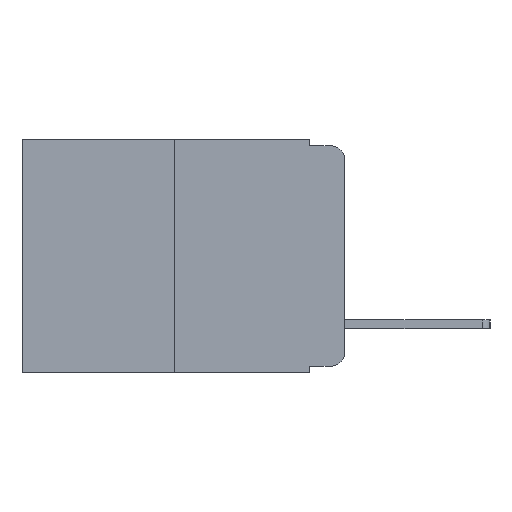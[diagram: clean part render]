
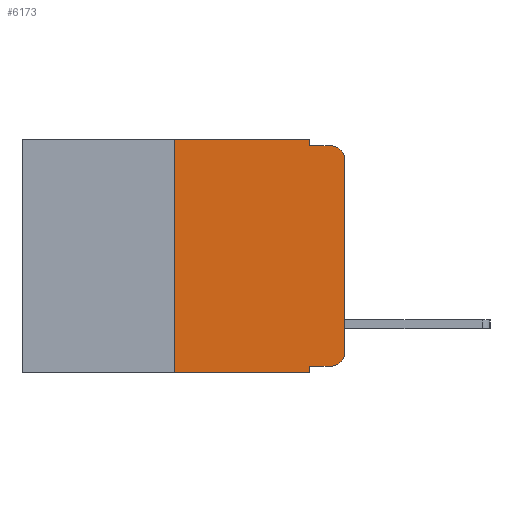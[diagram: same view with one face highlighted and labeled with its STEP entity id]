
A CAD part, left-side view. The second image highlights one B-rep face of the part: STEP entity #6173.
In plain terms, the highlighted planar face has unit normal (-1, 0, 0).
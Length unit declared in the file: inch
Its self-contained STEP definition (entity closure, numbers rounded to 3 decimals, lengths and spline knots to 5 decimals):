
#895 = LINE ( 'NONE', #17830, #14827 ) ;
#1033 = ORIENTED_EDGE ( 'NONE', *, *, #17482, .F. ) ;
#1414 = VERTEX_POINT ( 'NONE', #18648 ) ;
#1776 = EDGE_LOOP ( 'NONE', ( #20185, #4307, #9606, #12827, #3194, #1033, #14149, #10768, #17269, #14955 ) ) ;
#3194 = ORIENTED_EDGE ( 'NONE', *, *, #20132, .F. ) ;
#3628 = DIRECTION ( 'NONE',  ( -1., 0., 0. ) ) ;
#3835 = DIRECTION ( 'NONE',  ( 0., -1., 0. ) ) ;
#4049 = CARTESIAN_POINT ( 'NONE',  ( 0., 0.051, 0. ) ) ;
#4067 = VERTEX_POINT ( 'NONE', #14452 ) ;
#4307 = ORIENTED_EDGE ( 'NONE', *, *, #20642, .T. ) ;
#4696 = VERTEX_POINT ( 'NONE', #22398 ) ;
#4763 = CARTESIAN_POINT ( 'NONE',  ( 0., 0.473, 0. ) ) ;
#5583 = DIRECTION ( 'NONE',  ( 0., 0., 1. ) ) ;
#5677 = VECTOR ( 'NONE', #7814, 39.37008 ) ;
#5726 = CARTESIAN_POINT ( 'NONE',  ( 0., 0.02, -0.03 ) ) ;
#5925 = CARTESIAN_POINT ( 'NONE',  ( 0., 0.051, -0.01 ) ) ;
#6173 = ADVANCED_FACE ( 'NONE', ( #21610 ), #21680, .F. ) ;
#6362 = CARTESIAN_POINT ( 'NONE',  ( 0., 0.051, 0. ) ) ;
#6380 = AXIS2_PLACEMENT_3D ( 'NONE', #14364, #3628, #16050 ) ;
#6572 = VECTOR ( 'NONE', #11750, 39.37008 ) ;
#7038 = VECTOR ( 'NONE', #21076, 39.37008 ) ;
#7577 = DIRECTION ( 'NONE',  ( 0., 0., -1. ) ) ;
#7814 = DIRECTION ( 'NONE',  ( 0., 0., -1. ) ) ;
#8091 = CARTESIAN_POINT ( 'NONE',  ( 0., 0.25, 0. ) ) ;
#8227 = VERTEX_POINT ( 'NONE', #16112 ) ;
#8401 = CIRCLE ( 'NONE', #6380, 0.02 ) ;
#9240 = DIRECTION ( 'NONE',  ( 0., -1., 0. ) ) ;
#9606 = ORIENTED_EDGE ( 'NONE', *, *, #19578, .F. ) ;
#9903 = VECTOR ( 'NONE', #3835, 39.37008 ) ;
#10152 = CARTESIAN_POINT ( 'NONE',  ( 0., 0.051, 0. ) ) ;
#10335 = LINE ( 'NONE', #11025, #13747 ) ;
#10343 = CARTESIAN_POINT ( 'NONE',  ( 0., 0.473, 0. ) ) ;
#10585 = LINE ( 'NONE', #4049, #5677 ) ;
#10768 = ORIENTED_EDGE ( 'NONE', *, *, #16415, .F. ) ;
#11025 = CARTESIAN_POINT ( 'NONE',  ( 0., 0.25, 0. ) ) ;
#11102 = EDGE_CURVE ( 'NONE', #8227, #12383, #14393, .T. ) ;
#11103 = CARTESIAN_POINT ( 'NONE',  ( 0., 0.051, -0.01 ) ) ;
#11256 = DIRECTION ( 'NONE',  ( 0., -1., 0. ) ) ;
#11750 = DIRECTION ( 'NONE',  ( 0., 0., -1. ) ) ;
#12000 = DIRECTION ( 'NONE',  ( 1., 0., 0. ) ) ;
#12383 = VERTEX_POINT ( 'NONE', #18413 ) ;
#12389 = LINE ( 'NONE', #11103, #16309 ) ;
#12827 = ORIENTED_EDGE ( 'NONE', *, *, #18543, .F. ) ;
#13037 = EDGE_CURVE ( 'NONE', #4696, #4067, #8401, .T. ) ;
#13095 = AXIS2_PLACEMENT_3D ( 'NONE', #5726, #17793, #7577 ) ;
#13642 = DIRECTION ( 'NONE',  ( 0., -1., 0. ) ) ;
#13747 = VECTOR ( 'NONE', #5583, 39.37008 ) ;
#13942 = LINE ( 'NONE', #10343, #19256 ) ;
#14149 = ORIENTED_EDGE ( 'NONE', *, *, #11102, .T. ) ;
#14364 = CARTESIAN_POINT ( 'NONE',  ( 0., 0.02, -0.313 ) ) ;
#14393 = LINE ( 'NONE', #22484, #9903 ) ;
#14452 = CARTESIAN_POINT ( 'NONE',  ( 0., 0., -0.313 ) ) ;
#14751 = VERTEX_POINT ( 'NONE', #10152 ) ;
#14827 = VECTOR ( 'NONE', #11256, 39.37008 ) ;
#14843 = AXIS2_PLACEMENT_3D ( 'NONE', #4763, #12000, #18508 ) ;
#14955 = ORIENTED_EDGE ( 'NONE', *, *, #13037, .T. ) ;
#15212 = VERTEX_POINT ( 'NONE', #20862 ) ;
#15319 = EDGE_CURVE ( 'NONE', #22391, #4696, #895, .T. ) ;
#15381 = VERTEX_POINT ( 'NONE', #5925 ) ;
#15568 = VERTEX_POINT ( 'NONE', #8091 ) ;
#15735 = LINE ( 'NONE', #19416, #7038 ) ;
#16012 = CIRCLE ( 'NONE', #13095, 0.02 ) ;
#16050 = DIRECTION ( 'NONE',  ( 0., 0., -1. ) ) ;
#16112 = CARTESIAN_POINT ( 'NONE',  ( 0., 0.25, -0.343 ) ) ;
#16309 = VECTOR ( 'NONE', #9240, 39.37008 ) ;
#16415 = EDGE_CURVE ( 'NONE', #22391, #12383, #20059, .T. ) ;
#17269 = ORIENTED_EDGE ( 'NONE', *, *, #15319, .T. ) ;
#17482 = EDGE_CURVE ( 'NONE', #8227, #15568, #10335, .T. ) ;
#17793 = DIRECTION ( 'NONE',  ( -1., 0., 0. ) ) ;
#17830 = CARTESIAN_POINT ( 'NONE',  ( 0., 0.051, -0.333 ) ) ;
#18413 = CARTESIAN_POINT ( 'NONE',  ( 0., 0.051, -0.343 ) ) ;
#18508 = DIRECTION ( 'NONE',  ( 0., 0., -1. ) ) ;
#18543 = EDGE_CURVE ( 'NONE', #14751, #15381, #10585, .T. ) ;
#18648 = CARTESIAN_POINT ( 'NONE',  ( 0., 0.02, -0.01 ) ) ;
#18859 = CARTESIAN_POINT ( 'NONE',  ( 0., 0.051, -0.333 ) ) ;
#19256 = VECTOR ( 'NONE', #13642, 39.37008 ) ;
#19416 = CARTESIAN_POINT ( 'NONE',  ( 0., 0., 0. ) ) ;
#19578 = EDGE_CURVE ( 'NONE', #15381, #1414, #12389, .T. ) ;
#20059 = LINE ( 'NONE', #6362, #6572 ) ;
#20132 = EDGE_CURVE ( 'NONE', #15568, #14751, #13942, .T. ) ;
#20185 = ORIENTED_EDGE ( 'NONE', *, *, #21709, .T. ) ;
#20642 = EDGE_CURVE ( 'NONE', #15212, #1414, #16012, .T. ) ;
#20862 = CARTESIAN_POINT ( 'NONE',  ( 0., 0., -0.03 ) ) ;
#21076 = DIRECTION ( 'NONE',  ( 0., 0., 1. ) ) ;
#21610 = FACE_OUTER_BOUND ( 'NONE', #1776, .T. ) ;
#21680 = PLANE ( 'NONE',  #14843 ) ;
#21709 = EDGE_CURVE ( 'NONE', #4067, #15212, #15735, .T. ) ;
#22391 = VERTEX_POINT ( 'NONE', #18859 ) ;
#22398 = CARTESIAN_POINT ( 'NONE',  ( 0., 0.02, -0.333 ) ) ;
#22484 = CARTESIAN_POINT ( 'NONE',  ( 0., 0.473, -0.343 ) ) ;
